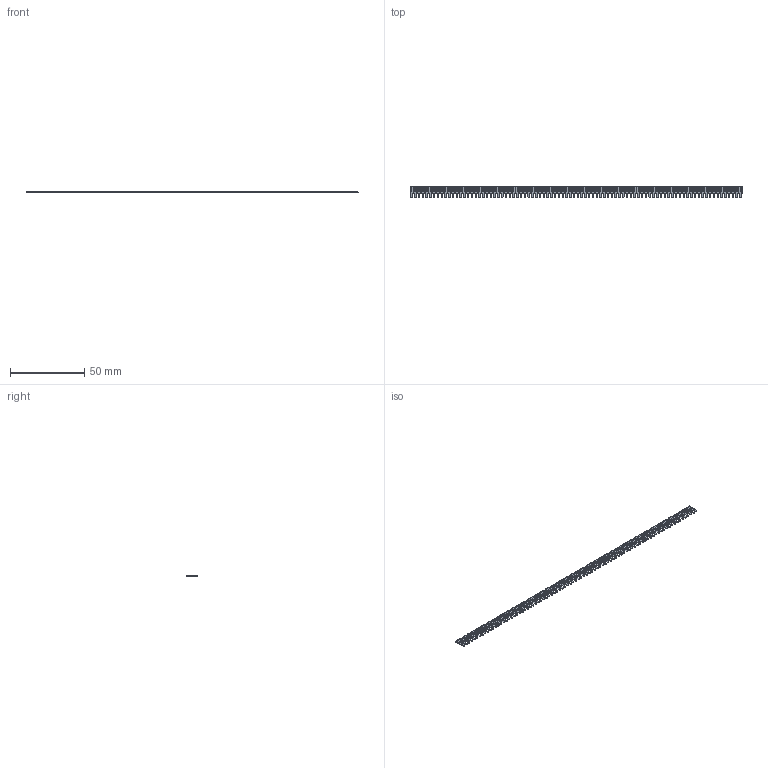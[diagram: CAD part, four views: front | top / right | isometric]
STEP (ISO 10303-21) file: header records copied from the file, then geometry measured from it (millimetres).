
FILE_DESCRIPTION (( 'STEP AP203' ), '1' );
FILE_NAME ('103-088-253-100.STEP', '2020-04-16T17:00:24', ( '' ), ( '' ), 'SwSTEP 2.0', 'SolidWorks 2016', '' );
FILE_SCHEMA (( 'CONFIG_CONTROL_DESIGN' ));
Length unit declared in the file: inch
Products named in the file (2): 103-088-253-100; 100-290-001_100-290-253
Assembly tree (88 placements, depth 2):
  103-088-253-100
    100-290-001_100-290-253  x88
Bounding box: 223.01 x 7.62 x 0.51 mm (x, y, z)
Volume: 485.5 mm3; surface area: 3027.8 mm2
Topology: 88 solids, 88 shells, 1760 faces, 4752 edges, 3168 vertices
Faces by surface type: plane 1672, cylinder 88
Entity records: 3604 total; most frequent: DIRECTION 278, CARTESIAN_POINT 201, COORDINATED_UNIVERSAL_TIME_OFFSET 186, LOCAL_TIME 186, CALENDAR_DATE 186, DATE_AND_TIME 186, AXIS2_PLACEMENT_3D 113, ORIENTED_EDGE 108
